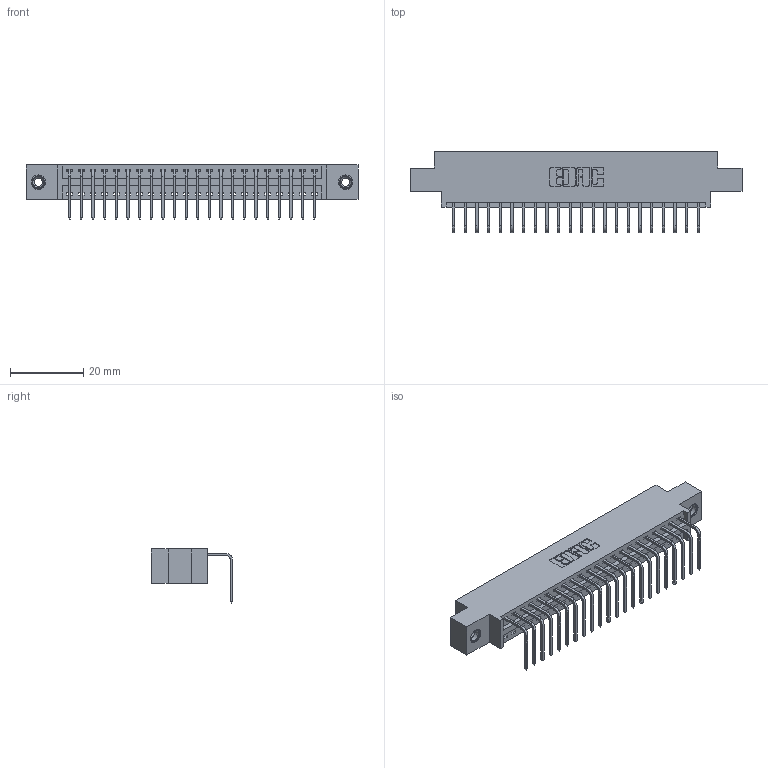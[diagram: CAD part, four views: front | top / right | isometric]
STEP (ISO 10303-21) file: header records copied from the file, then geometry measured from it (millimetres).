
FILE_DESCRIPTION (( 'STEP AP203' ), '1' );
FILE_NAME ('396-022-558-608.STEP', '2019-11-01T06:19:30', ( '' ), ( '' ), 'SwSTEP 2.0', 'SolidWorks 2016', '' );
FILE_SCHEMA (( 'CONFIG_CONTROL_DESIGN' ));
Length unit declared in the file: inch
Products named in the file (4): 396-022-558-608; 346 Part_0.170 Offset - 0.156 Dia-TI; 345-292-001_558 Tail - 2; 345-250-001_345-250-003-102
Assembly tree (25 placements, depth 2):
  396-022-558-608
    346 Part_0.170 Offset - 0.156 Dia-TI
    345-292-001_558 Tail - 2  x22
    345-250-001_345-250-003-102  x2
Bounding box: 90.42 x 22.16 x 14.73 mm (x, y, z)
Volume: 8430 mm3; surface area: 10940 mm2
Topology: 25 solids, 25 shells, 1506 faces, 4481 edges, 2950 vertices
Faces by surface type: plane 1036, cylinder 454, cone 12, torus 4
Entity records: 17748 total; most frequent: CARTESIAN_POINT 3033, ORIENTED_EDGE 2982, DIRECTION 2725, EDGE_CURVE 1491, VECTOR 1251, LINE 1251, VERTEX_POINT 988, AXIS2_PLACEMENT_3D 737
